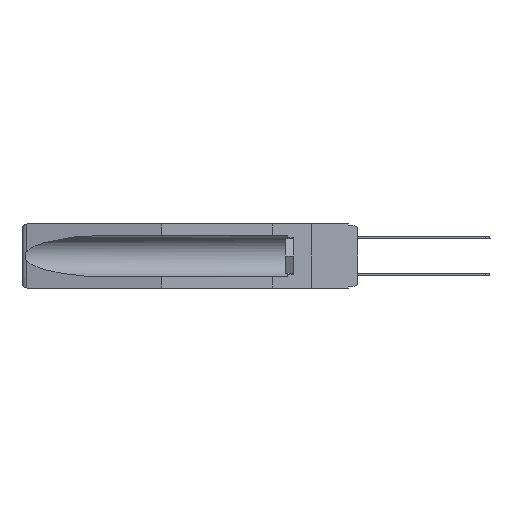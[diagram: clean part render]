
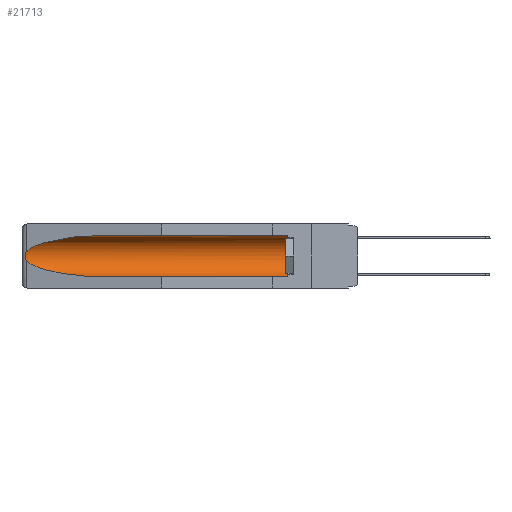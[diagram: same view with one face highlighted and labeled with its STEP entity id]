
A CAD part, left-side view. The second image highlights one B-rep face of the part: STEP entity #21713.
In plain terms, the highlighted cylindrical face has radius 2.857 mm (diameter 5.715 mm), a partial arc.
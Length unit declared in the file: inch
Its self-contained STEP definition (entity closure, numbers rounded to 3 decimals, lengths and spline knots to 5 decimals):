
#254 = ORIENTED_EDGE ( 'NONE', *, *, #8671, .F. ) ;
#700 = DIRECTION ( 'NONE',  ( 0., 0., 1. ) ) ;
#703 = DIRECTION ( 'NONE',  ( 0., 1., 0. ) ) ;
#1136 = ORIENTED_EDGE ( 'NONE', *, *, #21469, .T. ) ;
#1242 = CARTESIAN_POINT ( 'NONE',  ( 0.2673, 1.5327, -0.16383 ) ) ;
#1306 = CARTESIAN_POINT ( 'NONE',  ( 0.2675, 1.53308, -0.16763 ) ) ;
#1609 = CARTESIAN_POINT ( 'NONE',  ( 0.155, 0.126, -0.1715 ) ) ;
#1772 = VERTEX_POINT ( 'NONE', #3090 ) ;
#2137 = ORIENTED_EDGE ( 'NONE', *, *, #20564, .T. ) ;
#2978 = EDGE_CURVE ( 'NONE', #15704, #9856, #15598, .T. ) ;
#3090 = CARTESIAN_POINT ( 'NONE',  ( 0.155, 1.07973, -0.059 ) ) ;
#3498 = CARTESIAN_POINT ( 'NONE',  ( 0.25451, 1.48313, -0.09465 ) ) ;
#4218 = EDGE_CURVE ( 'NONE', #16382, #13891, #7640, .T. ) ;
#4540 = FACE_OUTER_BOUND ( 'NONE', #15497, .T. ) ;
#4801 = CARTESIAN_POINT ( 'NONE',  ( 0.155, -0.30754, -0.1715 ) ) ;
#4978 = ORIENTED_EDGE ( 'NONE', *, *, #4218, .T. ) ;
#6522 = DIRECTION ( 'NONE',  ( 0., 0., 1. ) ) ;
#6786 = CARTESIAN_POINT ( 'NONE',  ( 0.26537, 1.52718, -0.19328 ) ) ;
#6896 = ORIENTED_EDGE ( 'NONE', *, *, #21028, .T. ) ;
#7150 = CARTESIAN_POINT ( 'NONE',  ( 0.155, 0.126, -0.059 ) ) ;
#7640 =( BOUNDED_CURVE ( )  B_SPLINE_CURVE ( 3, ( #6786, #13814, #10221, #18968 ),
 .UNSPECIFIED., .F., .T. ) 
 B_SPLINE_CURVE_WITH_KNOTS ( ( 4, 4 ),
 ( 0.1948, 1.5708 ),
 .UNSPECIFIED. ) 
 CURVE ( )  GEOMETRIC_REPRESENTATION_ITEM ( )  RATIONAL_B_SPLINE_CURVE ( ( 1., 0.848, 0.848, 1. ) ) 
 REPRESENTATION_ITEM ( '' )  );
#7704 = CARTESIAN_POINT ( 'NONE',  ( 0.155, 0.126, -0.284 ) ) ;
#8348 = CARTESIAN_POINT ( 'NONE',  ( 0.26655, 1.53094, -0.18657 ) ) ;
#8470 = DIRECTION ( 'NONE',  ( 0., 1., 0. ) ) ;
#8671 = EDGE_CURVE ( 'NONE', #15704, #13891, #18686, .T. ) ;
#9856 = VERTEX_POINT ( 'NONE', #7150 ) ;
#10221 = CARTESIAN_POINT ( 'NONE',  ( 0.21114, 1.30732, -0.284 ) ) ;
#10620 = VECTOR ( 'NONE', #18022, 39.37008 ) ;
#11449 = CARTESIAN_POINT ( 'NONE',  ( 0.2673, 1.53269, -0.17917 ) ) ;
#11524 = CARTESIAN_POINT ( 'NONE',  ( 0.26654, 1.53092, -0.15636 ) ) ;
#11581 = CARTESIAN_POINT ( 'NONE',  ( 0.26537, 1.52718, -0.14972 ) ) ;
#11684 = CARTESIAN_POINT ( 'NONE',  ( 0.26537, 1.52718, -0.14972 ) ) ;
#12011 = CARTESIAN_POINT ( 'NONE',  ( 0.26537, 1.52718, -0.14972 ) ) ;
#12873 = CARTESIAN_POINT ( 'NONE',  ( 0.155, -0.30754, -0.059 ) ) ;
#13099 = CYLINDRICAL_SURFACE ( 'NONE', #16539, 0.1125 ) ;
#13459 = CARTESIAN_POINT ( 'NONE',  ( 0.21114, 1.30732, -0.059 ) ) ;
#13610 = CARTESIAN_POINT ( 'NONE',  ( 0.155, 1.07973, -0.059 ) ) ;
#13788 = DIRECTION ( 'NONE',  ( 0., -1., 0. ) ) ;
#13814 = CARTESIAN_POINT ( 'NONE',  ( 0.25451, 1.48313, -0.24835 ) ) ;
#13891 = VERTEX_POINT ( 'NONE', #17545 ) ;
#15124 = CARTESIAN_POINT ( 'NONE',  ( 0.26597, 1.5296, -0.19026 ) ) ;
#15172 = VERTEX_POINT ( 'NONE', #11581 ) ;
#15218 = VECTOR ( 'NONE', #703, 39.37008 ) ;
#15497 = EDGE_LOOP ( 'NONE', ( #2137, #6896, #4978, #254, #17328, #1136 ) ) ;
#15598 = CIRCLE ( 'NONE', #19334, 0.1125 ) ;
#15704 = VERTEX_POINT ( 'NONE', #7704 ) ;
#16382 = VERTEX_POINT ( 'NONE', #21429 ) ;
#16539 = AXIS2_PLACEMENT_3D ( 'NONE', #4801, #8470, #6522 ) ;
#17328 = ORIENTED_EDGE ( 'NONE', *, *, #2978, .T. ) ;
#17373 = LINE ( 'NONE', #12873, #15218 ) ;
#17545 = CARTESIAN_POINT ( 'NONE',  ( 0.155, 1.07973, -0.284 ) ) ;
#18022 = DIRECTION ( 'NONE',  ( 0., 1., 0. ) ) ;
#18308 =( BOUNDED_CURVE ( )  B_SPLINE_CURVE ( 3, ( #13610, #13459, #3498, #12011 ),
 .UNSPECIFIED., .F., .F. ) 
 B_SPLINE_CURVE_WITH_KNOTS ( ( 4, 4 ),
 ( 4.71239, 6.08839 ),
 .UNSPECIFIED. ) 
 CURVE ( )  GEOMETRIC_REPRESENTATION_ITEM ( )  RATIONAL_B_SPLINE_CURVE ( ( 1., 0.848, 0.848, 1. ) ) 
 REPRESENTATION_ITEM ( '' )  );
#18504 = CARTESIAN_POINT ( 'NONE',  ( 0.2675, 1.53308, -0.17534 ) ) ;
#18686 = LINE ( 'NONE', #19828, #10620 ) ;
#18968 = CARTESIAN_POINT ( 'NONE',  ( 0.155, 1.07973, -0.284 ) ) ;
#19334 = AXIS2_PLACEMENT_3D ( 'NONE', #1609, #13788, #700 ) ;
#19828 = CARTESIAN_POINT ( 'NONE',  ( 0.155, -0.30754, -0.284 ) ) ;
#19962 = B_SPLINE_CURVE_WITH_KNOTS ( 'NONE', 3,
 ( #11684, #21893, #11524, #1242, #1306, #18504, #11449, #8348, #15124, #20227 ),
 .UNSPECIFIED., .F., .F.,
 ( 4, 2, 2, 2, 4 ),
 ( 0., 0.00029, 0.00058, 0.00087, 0.00117 ),
 .UNSPECIFIED. ) ;
#20227 = CARTESIAN_POINT ( 'NONE',  ( 0.26537, 1.52718, -0.19328 ) ) ;
#20564 = EDGE_CURVE ( 'NONE', #1772, #15172, #18308, .T. ) ;
#21028 = EDGE_CURVE ( 'NONE', #15172, #16382, #19962, .T. ) ;
#21429 = CARTESIAN_POINT ( 'NONE',  ( 0.26537, 1.52718, -0.19328 ) ) ;
#21469 = EDGE_CURVE ( 'NONE', #9856, #1772, #17373, .T. ) ;
#21713 = ADVANCED_FACE ( 'NONE', ( #4540 ), #13099, .F. ) ;
#21893 = CARTESIAN_POINT ( 'NONE',  ( 0.26597, 1.52961, -0.15275 ) ) ;
